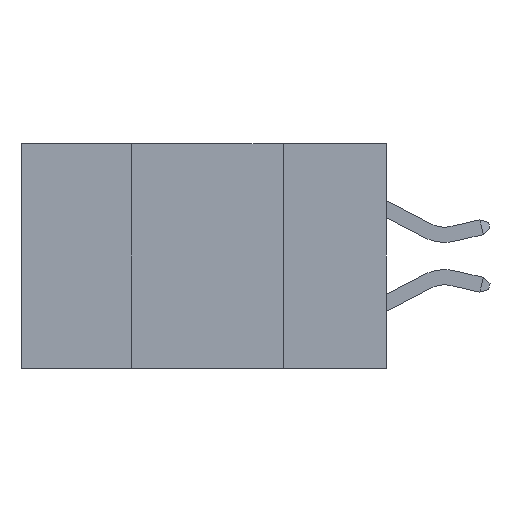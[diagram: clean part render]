
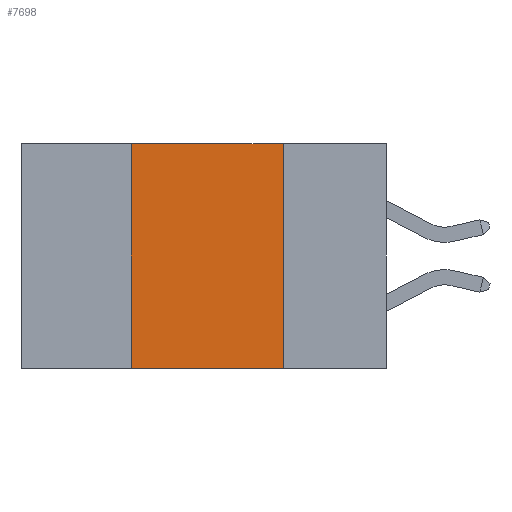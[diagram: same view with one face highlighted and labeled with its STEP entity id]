
A CAD part, left-side view. The second image highlights one B-rep face of the part: STEP entity #7698.
In plain terms, the highlighted planar face has unit normal (-1, 0, 0).
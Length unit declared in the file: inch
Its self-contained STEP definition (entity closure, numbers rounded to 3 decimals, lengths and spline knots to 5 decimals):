
#30 = CARTESIAN_POINT ( 'NONE',  ( 0., 0.17, -0.37 ) ) ;
#342 = CARTESIAN_POINT ( 'NONE',  ( 0., 0.17, 0. ) ) ;
#472 = DIRECTION ( 'NONE',  ( 0., -1., 0. ) ) ;
#842 = DIRECTION ( 'NONE',  ( 0., 0., -1. ) ) ;
#1224 = LINE ( 'NONE', #2666, #10834 ) ;
#1271 = CARTESIAN_POINT ( 'NONE',  ( 0., 0.42, -0.37 ) ) ;
#1835 = CARTESIAN_POINT ( 'NONE',  ( 0., 0.42, 0. ) ) ;
#2126 = EDGE_LOOP ( 'NONE', ( #6712, #2970, #4137, #9051 ) ) ;
#2666 = CARTESIAN_POINT ( 'NONE',  ( 0., 0.6, -0.37 ) ) ;
#2764 = DIRECTION ( 'NONE',  ( 0., -1., 0. ) ) ;
#2792 = CARTESIAN_POINT ( 'NONE',  ( 0., 0.6, 0. ) ) ;
#2970 = ORIENTED_EDGE ( 'NONE', *, *, #5541, .F. ) ;
#3087 = EDGE_CURVE ( 'NONE', #4883, #11759, #1224, .T. ) ;
#4137 = ORIENTED_EDGE ( 'NONE', *, *, #4322, .F. ) ;
#4322 = EDGE_CURVE ( 'NONE', #4883, #4578, #8960, .T. ) ;
#4578 = VERTEX_POINT ( 'NONE', #1835 ) ;
#4883 = VERTEX_POINT ( 'NONE', #1271 ) ;
#5035 = VECTOR ( 'NONE', #472, 39.37008 ) ;
#5132 = VECTOR ( 'NONE', #5636, 39.37008 ) ;
#5422 = LINE ( 'NONE', #11155, #5132 ) ;
#5541 = EDGE_CURVE ( 'NONE', #4578, #9138, #9961, .T. ) ;
#5636 = DIRECTION ( 'NONE',  ( 0., 0., -1. ) ) ;
#6499 = DIRECTION ( 'NONE',  ( 1., 0., 0. ) ) ;
#6712 = ORIENTED_EDGE ( 'NONE', *, *, #9899, .F. ) ;
#7071 = CARTESIAN_POINT ( 'NONE',  ( 0., 0.42, -0.37 ) ) ;
#7083 = CARTESIAN_POINT ( 'NONE',  ( 0., 0.6, 0. ) ) ;
#7441 = FACE_OUTER_BOUND ( 'NONE', #2126, .T. ) ;
#7698 = ADVANCED_FACE ( 'NONE', ( #7441 ), #12004, .F. ) ;
#8960 = LINE ( 'NONE', #7071, #11383 ) ;
#9051 = ORIENTED_EDGE ( 'NONE', *, *, #3087, .T. ) ;
#9138 = VERTEX_POINT ( 'NONE', #342 ) ;
#9899 = EDGE_CURVE ( 'NONE', #9138, #11759, #5422, .T. ) ;
#9961 = LINE ( 'NONE', #7083, #5035 ) ;
#10834 = VECTOR ( 'NONE', #2764, 39.37008 ) ;
#11142 = AXIS2_PLACEMENT_3D ( 'NONE', #2792, #6499, #842 ) ;
#11155 = CARTESIAN_POINT ( 'NONE',  ( 0., 0.17, -0.37 ) ) ;
#11383 = VECTOR ( 'NONE', #11600, 39.37008 ) ;
#11600 = DIRECTION ( 'NONE',  ( 0., 0., 1. ) ) ;
#11759 = VERTEX_POINT ( 'NONE', #30 ) ;
#12004 = PLANE ( 'NONE',  #11142 ) ;
